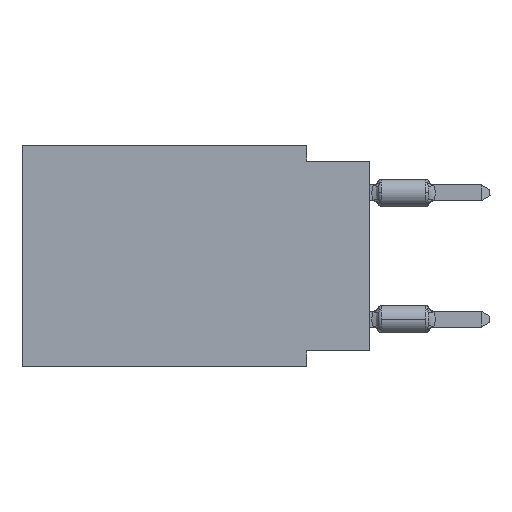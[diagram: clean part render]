
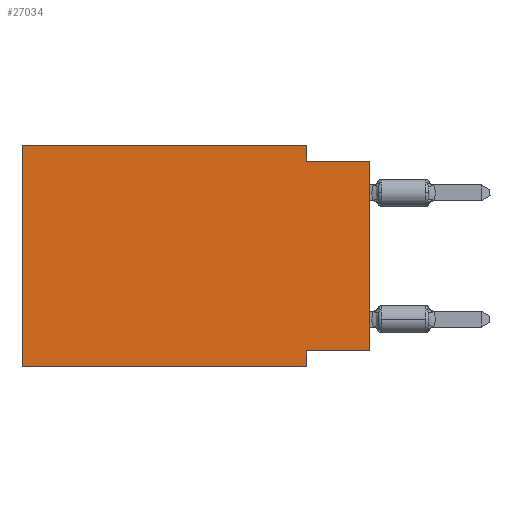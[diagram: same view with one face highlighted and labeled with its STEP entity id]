
A CAD part, left-side view. The second image highlights one B-rep face of the part: STEP entity #27034.
In plain terms, the highlighted planar face has unit normal (-1, 0, 0).
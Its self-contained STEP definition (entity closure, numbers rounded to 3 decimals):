
#1151 = LINE ( 'NONE', #40024, #5609 ) ;
#1530 = CARTESIAN_POINT ( 'NONE',  ( 0., 13.97, 0. ) ) ;
#2311 = ORIENTED_EDGE ( 'NONE', *, *, #10808, .F. ) ;
#4556 = AXIS2_PLACEMENT_3D ( 'NONE', #28097, #4832, #8925 ) ;
#4832 = DIRECTION ( 'NONE',  ( 1., 0., 0. ) ) ;
#5609 = VECTOR ( 'NONE', #5751, 1000. ) ;
#5693 = VERTEX_POINT ( 'NONE', #5792 ) ;
#5751 = DIRECTION ( 'NONE',  ( 0., 1., 0. ) ) ;
#5776 = CARTESIAN_POINT ( 'NONE',  ( 0., 13.97, -8.89 ) ) ;
#5792 = CARTESIAN_POINT ( 'NONE',  ( 0., 2.54, 0. ) ) ;
#5872 = VERTEX_POINT ( 'NONE', #6545 ) ;
#6545 = CARTESIAN_POINT ( 'NONE',  ( 0., 2.54, -8.255 ) ) ;
#7413 = DIRECTION ( 'NONE',  ( 0., 0., 1. ) ) ;
#8925 = DIRECTION ( 'NONE',  ( 0., 0., -1. ) ) ;
#9347 = ORIENTED_EDGE ( 'NONE', *, *, #38342, .F. ) ;
#10808 = EDGE_CURVE ( 'NONE', #40139, #14350, #41950, .T. ) ;
#11496 = CARTESIAN_POINT ( 'NONE',  ( 0., 13.97, -8.89 ) ) ;
#11845 = CARTESIAN_POINT ( 'NONE',  ( 0., 2.54, -8.89 ) ) ;
#11893 = VECTOR ( 'NONE', #46379, 1000. ) ;
#12845 = LINE ( 'NONE', #36344, #31477 ) ;
#14210 = LINE ( 'NONE', #5776, #27191 ) ;
#14350 = VERTEX_POINT ( 'NONE', #24269 ) ;
#14959 = CARTESIAN_POINT ( 'NONE',  ( 0., 2.54, -8.89 ) ) ;
#18823 = CARTESIAN_POINT ( 'NONE',  ( 0., 2.54, 0. ) ) ;
#19565 = CARTESIAN_POINT ( 'NONE',  ( 0., 2.54, -0.635 ) ) ;
#19645 = ORIENTED_EDGE ( 'NONE', *, *, #45827, .F. ) ;
#21131 = DIRECTION ( 'NONE',  ( 0., -1., 0. ) ) ;
#21190 = PLANE ( 'NONE',  #4556 ) ;
#22985 = VERTEX_POINT ( 'NONE', #11496 ) ;
#23541 = LINE ( 'NONE', #1530, #49526 ) ;
#23661 = ORIENTED_EDGE ( 'NONE', *, *, #41813, .F. ) ;
#23667 = LINE ( 'NONE', #18823, #38162 ) ;
#23700 = ORIENTED_EDGE ( 'NONE', *, *, #45102, .F. ) ;
#24254 = CARTESIAN_POINT ( 'NONE',  ( 0., 0., -8.255 ) ) ;
#24269 = CARTESIAN_POINT ( 'NONE',  ( 0., 0., -0.635 ) ) ;
#26597 = CARTESIAN_POINT ( 'NONE',  ( 0., 0., -0.635 ) ) ;
#26991 = DIRECTION ( 'NONE',  ( 0., 0., -1. ) ) ;
#27034 = ADVANCED_FACE ( 'NONE', ( #40640 ), #21190, .F. ) ;
#27163 = VERTEX_POINT ( 'NONE', #42155 ) ;
#27191 = VECTOR ( 'NONE', #21131, 1000. ) ;
#28097 = CARTESIAN_POINT ( 'NONE',  ( 0., 13.97, 0. ) ) ;
#30130 = ORIENTED_EDGE ( 'NONE', *, *, #49947, .T. ) ;
#31477 = VECTOR ( 'NONE', #47357, 1000. ) ;
#34507 = DIRECTION ( 'NONE',  ( 0., -1., 0. ) ) ;
#35267 = CARTESIAN_POINT ( 'NONE',  ( 0., 13.97, 0. ) ) ;
#35348 = LINE ( 'NONE', #11845, #11893 ) ;
#36344 = CARTESIAN_POINT ( 'NONE',  ( 0., 0., 0. ) ) ;
#37252 = VERTEX_POINT ( 'NONE', #24254 ) ;
#37909 = VERTEX_POINT ( 'NONE', #14959 ) ;
#38162 = VECTOR ( 'NONE', #26991, 1000. ) ;
#38342 = EDGE_CURVE ( 'NONE', #22985, #27163, #42460, .T. ) ;
#38672 = VECTOR ( 'NONE', #7413, 1000. ) ;
#39090 = EDGE_CURVE ( 'NONE', #22985, #37909, #14210, .T. ) ;
#40024 = CARTESIAN_POINT ( 'NONE',  ( 0., 0., -8.255 ) ) ;
#40139 = VERTEX_POINT ( 'NONE', #19565 ) ;
#40346 = VECTOR ( 'NONE', #34507, 1000. ) ;
#40640 = FACE_OUTER_BOUND ( 'NONE', #41487, .T. ) ;
#41487 = EDGE_LOOP ( 'NONE', ( #30130, #2311, #19645, #23700, #9347, #46075, #23661, #48681 ) ) ;
#41813 = EDGE_CURVE ( 'NONE', #5872, #37909, #35348, .T. ) ;
#41950 = LINE ( 'NONE', #26597, #40346 ) ;
#42155 = CARTESIAN_POINT ( 'NONE',  ( 0., 13.97, 0. ) ) ;
#42460 = LINE ( 'NONE', #35267, #38672 ) ;
#45102 = EDGE_CURVE ( 'NONE', #27163, #5693, #23541, .T. ) ;
#45827 = EDGE_CURVE ( 'NONE', #5693, #40139, #23667, .T. ) ;
#46075 = ORIENTED_EDGE ( 'NONE', *, *, #39090, .T. ) ;
#46379 = DIRECTION ( 'NONE',  ( 0., 0., -1. ) ) ;
#47215 = EDGE_CURVE ( 'NONE', #37252, #5872, #1151, .T. ) ;
#47357 = DIRECTION ( 'NONE',  ( 0., 0., 1. ) ) ;
#48584 = DIRECTION ( 'NONE',  ( 0., -1., 0. ) ) ;
#48681 = ORIENTED_EDGE ( 'NONE', *, *, #47215, .F. ) ;
#49526 = VECTOR ( 'NONE', #48584, 1000. ) ;
#49947 = EDGE_CURVE ( 'NONE', #37252, #14350, #12845, .T. ) ;
